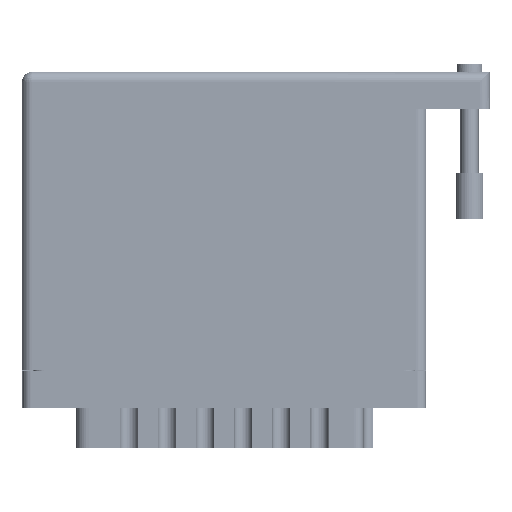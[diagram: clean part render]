
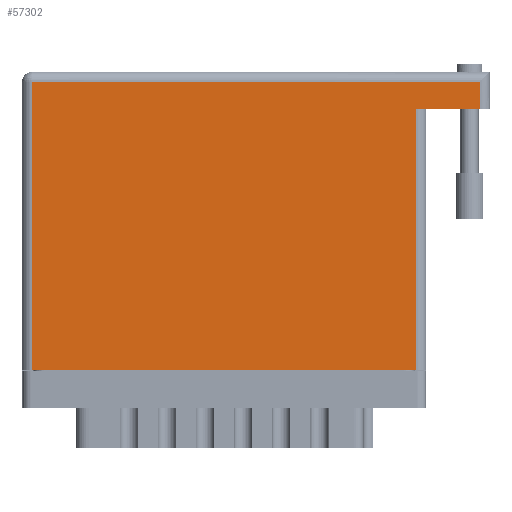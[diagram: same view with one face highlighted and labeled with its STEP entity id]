
A CAD part, front view. The second image highlights one B-rep face of the part: STEP entity #57302.
In plain terms, the highlighted face is planar.
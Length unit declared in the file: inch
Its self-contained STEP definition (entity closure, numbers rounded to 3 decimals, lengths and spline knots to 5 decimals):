
#5919 = FACE_OUTER_BOUND ( 'NONE', #64612, .T. ) ;
#11416 = VECTOR ( 'NONE', #35214, 39.37008 ) ;
#12251 = EDGE_CURVE ( 'NONE', #41542, #88789, #64215, .T. ) ;
#12572 = CARTESIAN_POINT ( 'NONE',  ( 0., 1.96, 0. ) ) ;
#13260 = ORIENTED_EDGE ( 'NONE', *, *, #19568, .T. ) ;
#13760 = CARTESIAN_POINT ( 'NONE',  ( 0.07, 1.96, 0. ) ) ;
#13815 = DIRECTION ( 'NONE',  ( 0., 1., 0. ) ) ;
#16735 = CARTESIAN_POINT ( 'NONE',  ( 0.07, 0., 0. ) ) ;
#17162 = PLANE ( 'NONE',  #81857 ) ;
#17875 = CARTESIAN_POINT ( 'NONE',  ( 2.685, 0., 0. ) ) ;
#19568 = EDGE_CURVE ( 'NONE', #73933, #26355, #73068, .T. ) ;
#21302 = EDGE_CURVE ( 'NONE', #81206, #63722, #63760, .T. ) ;
#25293 = DIRECTION ( 'NONE',  ( 0., 0., -1. ) ) ;
#26355 = VERTEX_POINT ( 'NONE', #77665 ) ;
#26899 = EDGE_CURVE ( 'NONE', #63722, #41542, #56311, .T. ) ;
#29560 = EDGE_CURVE ( 'NONE', #81206, #26355, #95770, .T. ) ;
#34570 = CARTESIAN_POINT ( 'NONE',  ( 2.685, 1.774, 0. ) ) ;
#35214 = DIRECTION ( 'NONE',  ( 0., 1., 0. ) ) ;
#37166 = CARTESIAN_POINT ( 'NONE',  ( 0., 0., 0. ) ) ;
#37482 = VECTOR ( 'NONE', #63220, 39.37008 ) ;
#40210 = CARTESIAN_POINT ( 'NONE',  ( 3.12, 1.96, 0. ) ) ;
#41542 = VERTEX_POINT ( 'NONE', #13760 ) ;
#41733 = ORIENTED_EDGE ( 'NONE', *, *, #26899, .T. ) ;
#44653 = DIRECTION ( 'NONE',  ( 1., 0., 0. ) ) ;
#45339 = VECTOR ( 'NONE', #44653, 39.37008 ) ;
#46028 = DIRECTION ( 'NONE',  ( -1., 0., 0. ) ) ;
#49594 = DIRECTION ( 'NONE',  ( -1., 0., 0. ) ) ;
#51628 = VECTOR ( 'NONE', #49594, 39.37008 ) ;
#53620 = ORIENTED_EDGE ( 'NONE', *, *, #21302, .T. ) ;
#54815 = VECTOR ( 'NONE', #68446, 39.37008 ) ;
#56311 = LINE ( 'NONE', #12572, #51628 ) ;
#57302 = ADVANCED_FACE ( 'NONE', ( #5919 ), #17162, .F. ) ;
#57810 = VECTOR ( 'NONE', #13815, 39.37008 ) ;
#63220 = DIRECTION ( 'NONE',  ( -1., 0., 0. ) ) ;
#63650 = CARTESIAN_POINT ( 'NONE',  ( 0.07, 0., 0. ) ) ;
#63722 = VERTEX_POINT ( 'NONE', #40210 ) ;
#63760 = LINE ( 'NONE', #65265, #57810 ) ;
#64215 = LINE ( 'NONE', #16735, #54815 ) ;
#64612 = EDGE_LOOP ( 'NONE', ( #88507, #13260, #85673, #53620, #41733, #83695 ) ) ;
#65265 = CARTESIAN_POINT ( 'NONE',  ( 3.12, 2.03, 0. ) ) ;
#67134 = EDGE_CURVE ( 'NONE', #88789, #73933, #77925, .T. ) ;
#68446 = DIRECTION ( 'NONE',  ( 0., -1., 0. ) ) ;
#69508 = CARTESIAN_POINT ( 'NONE',  ( 0., 2.03, 0. ) ) ;
#73068 = LINE ( 'NONE', #34570, #11416 ) ;
#73933 = VERTEX_POINT ( 'NONE', #17875 ) ;
#77665 = CARTESIAN_POINT ( 'NONE',  ( 2.685, 1.774, 0. ) ) ;
#77925 = LINE ( 'NONE', #37166, #45339 ) ;
#78049 = CARTESIAN_POINT ( 'NONE',  ( 3.19, 1.774, 0. ) ) ;
#81206 = VERTEX_POINT ( 'NONE', #86018 ) ;
#81857 = AXIS2_PLACEMENT_3D ( 'NONE', #69508, #25293, #46028 ) ;
#83695 = ORIENTED_EDGE ( 'NONE', *, *, #12251, .T. ) ;
#85673 = ORIENTED_EDGE ( 'NONE', *, *, #29560, .F. ) ;
#86018 = CARTESIAN_POINT ( 'NONE',  ( 3.12, 1.774, 0. ) ) ;
#88507 = ORIENTED_EDGE ( 'NONE', *, *, #67134, .T. ) ;
#88789 = VERTEX_POINT ( 'NONE', #63650 ) ;
#95770 = LINE ( 'NONE', #78049, #37482 ) ;
